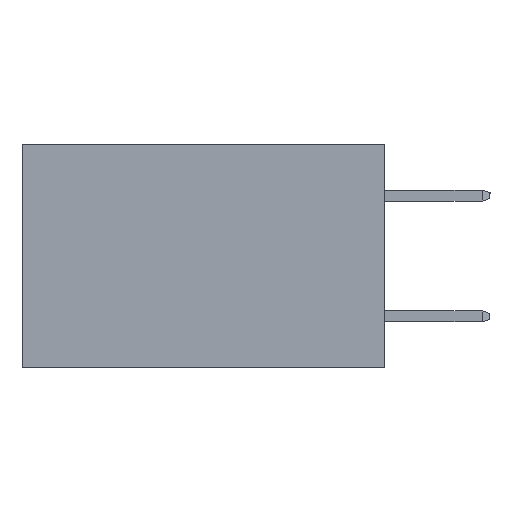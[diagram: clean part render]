
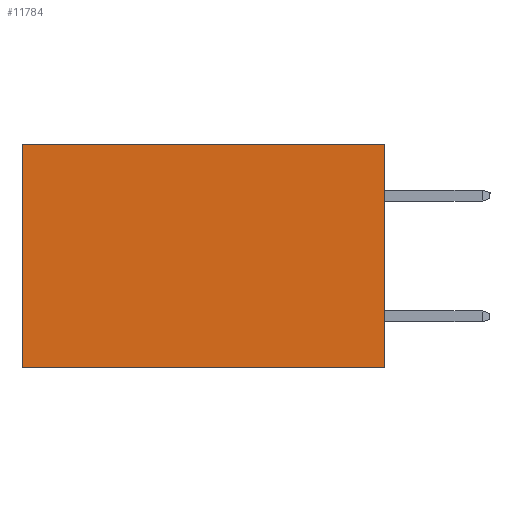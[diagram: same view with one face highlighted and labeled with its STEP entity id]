
A CAD part, left-side view. The second image highlights one B-rep face of the part: STEP entity #11784.
In plain terms, the highlighted planar face has unit normal (-1, 0, 0).
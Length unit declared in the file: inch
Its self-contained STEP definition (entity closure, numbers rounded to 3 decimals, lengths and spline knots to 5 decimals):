
#40 = ORIENTED_EDGE ( 'NONE', *, *, #12933, .F. ) ;
#78 = VECTOR ( 'NONE', #20130, 39.37008 ) ;
#325 = VECTOR ( 'NONE', #1841, 39.37008 ) ;
#326 = FACE_OUTER_BOUND ( 'NONE', #4983, .T. ) ;
#1094 = CARTESIAN_POINT ( 'NONE',  ( 0.2615, 0., -0.37 ) ) ;
#1206 = VERTEX_POINT ( 'NONE', #12191 ) ;
#1376 = VERTEX_POINT ( 'NONE', #20680 ) ;
#1607 = VECTOR ( 'NONE', #23097, 39.37008 ) ;
#1836 = LINE ( 'NONE', #3516, #78 ) ;
#1841 = DIRECTION ( 'NONE',  ( 0., 0., -1. ) ) ;
#2068 = LINE ( 'NONE', #11128, #325 ) ;
#2120 = DIRECTION ( 'NONE',  ( 0., 0., -1. ) ) ;
#3516 = CARTESIAN_POINT ( 'NONE',  ( 0.2615, 0., -0.37 ) ) ;
#4209 = ORIENTED_EDGE ( 'NONE', *, *, #23184, .T. ) ;
#4983 = EDGE_LOOP ( 'NONE', ( #4209, #40, #15243, #18024 ) ) ;
#8641 = LINE ( 'NONE', #20303, #1607 ) ;
#9449 = VECTOR ( 'NONE', #12293, 39.37008 ) ;
#11128 = CARTESIAN_POINT ( 'NONE',  ( 0.2615, 0.6, -0.37 ) ) ;
#11649 = EDGE_CURVE ( 'NONE', #15915, #1206, #8641, .T. ) ;
#11784 = ADVANCED_FACE ( 'NONE', ( #326 ), #22334, .F. ) ;
#12191 = CARTESIAN_POINT ( 'NONE',  ( 0.2615, 0.6, 0. ) ) ;
#12293 = DIRECTION ( 'NONE',  ( 0., 0., -1. ) ) ;
#12933 = EDGE_CURVE ( 'NONE', #1376, #20229, #1836, .T. ) ;
#14269 = CARTESIAN_POINT ( 'NONE',  ( 0.2615, 0.6, -0.37 ) ) ;
#15243 = ORIENTED_EDGE ( 'NONE', *, *, #18666, .F. ) ;
#15260 = CARTESIAN_POINT ( 'NONE',  ( 0.2615, 0., -0.37 ) ) ;
#15915 = VERTEX_POINT ( 'NONE', #23113 ) ;
#17734 = LINE ( 'NONE', #1094, #9449 ) ;
#18024 = ORIENTED_EDGE ( 'NONE', *, *, #11649, .T. ) ;
#18666 = EDGE_CURVE ( 'NONE', #15915, #1376, #17734, .T. ) ;
#20130 = DIRECTION ( 'NONE',  ( 0., 1., 0. ) ) ;
#20229 = VERTEX_POINT ( 'NONE', #14269 ) ;
#20303 = CARTESIAN_POINT ( 'NONE',  ( 0.2615, 0., 0. ) ) ;
#20680 = CARTESIAN_POINT ( 'NONE',  ( 0.2615, 0., -0.37 ) ) ;
#22227 = DIRECTION ( 'NONE',  ( 1., 0., 0. ) ) ;
#22334 = PLANE ( 'NONE',  #23545 ) ;
#23097 = DIRECTION ( 'NONE',  ( 0., 1., 0. ) ) ;
#23113 = CARTESIAN_POINT ( 'NONE',  ( 0.2615, 0., 0. ) ) ;
#23184 = EDGE_CURVE ( 'NONE', #1206, #20229, #2068, .T. ) ;
#23545 = AXIS2_PLACEMENT_3D ( 'NONE', #15260, #22227, #2120 ) ;
